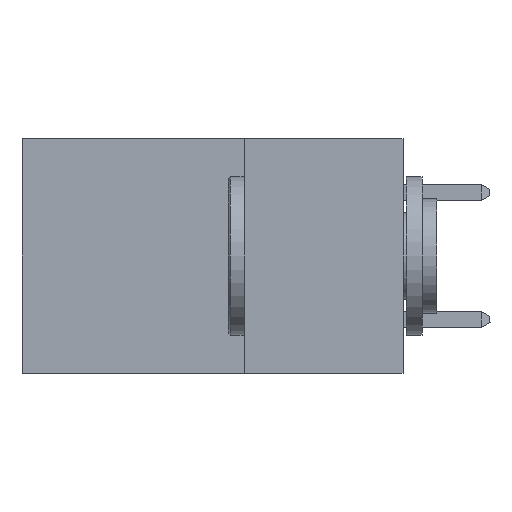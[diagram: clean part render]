
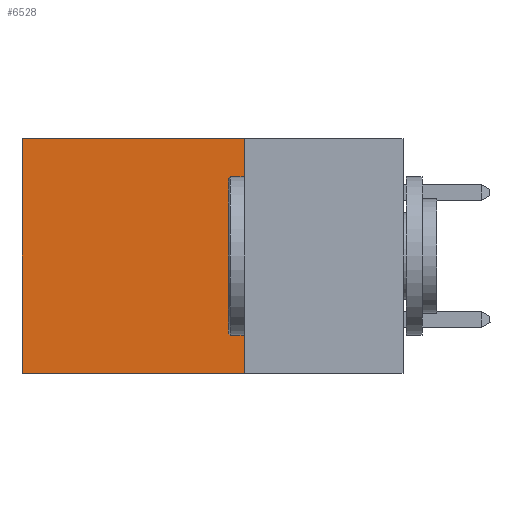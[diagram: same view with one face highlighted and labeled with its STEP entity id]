
A CAD part, left-side view. The second image highlights one B-rep face of the part: STEP entity #6528.
In plain terms, the highlighted planar face has unit normal (-1, 0, 0).
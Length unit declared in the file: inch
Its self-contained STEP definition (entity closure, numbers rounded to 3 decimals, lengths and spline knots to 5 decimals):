
#82 = FACE_OUTER_BOUND ( 'NONE', #4745, .T. ) ;
#235 = EDGE_CURVE ( 'NONE', #3854, #10123, #16813, .T. ) ;
#1263 = CARTESIAN_POINT ( 'NONE',  ( 0.2875, 0.25, 0. ) ) ;
#1335 = CARTESIAN_POINT ( 'NONE',  ( 0.2875, 0.25, 0. ) ) ;
#2133 = VERTEX_POINT ( 'NONE', #13537 ) ;
#3616 = EDGE_CURVE ( 'NONE', #3854, #2133, #17326, .T. ) ;
#3746 = CARTESIAN_POINT ( 'NONE',  ( 0.2875, 0.25, 0. ) ) ;
#3851 = DIRECTION ( 'NONE',  ( 0., 0., -1. ) ) ;
#3854 = VERTEX_POINT ( 'NONE', #3746 ) ;
#4299 = EDGE_CURVE ( 'NONE', #2133, #10515, #11146, .T. ) ;
#4745 = EDGE_LOOP ( 'NONE', ( #16329, #11081, #9070, #13059 ) ) ;
#5751 = DIRECTION ( 'NONE',  ( 0., 1., 0. ) ) ;
#6263 = VECTOR ( 'NONE', #3851, 39.37008 ) ;
#6358 = CARTESIAN_POINT ( 'NONE',  ( 0.2875, 0.25, -0.37 ) ) ;
#6528 = ADVANCED_FACE ( 'NONE', ( #82 ), #13390, .F. ) ;
#6806 = DIRECTION ( 'NONE',  ( 0., 0., -1. ) ) ;
#6993 = CARTESIAN_POINT ( 'NONE',  ( 0.2875, 0.25, 0. ) ) ;
#7622 = VECTOR ( 'NONE', #8741, 39.37008 ) ;
#8685 = LINE ( 'NONE', #14033, #15696 ) ;
#8741 = DIRECTION ( 'NONE',  ( 0., 0., -1. ) ) ;
#9070 = ORIENTED_EDGE ( 'NONE', *, *, #235, .F. ) ;
#9808 = CARTESIAN_POINT ( 'NONE',  ( 0.2875, 0.6, -0.37 ) ) ;
#10123 = VERTEX_POINT ( 'NONE', #6358 ) ;
#10144 = DIRECTION ( 'NONE',  ( 0., 1., 0. ) ) ;
#10317 = VECTOR ( 'NONE', #5751, 39.37008 ) ;
#10515 = VERTEX_POINT ( 'NONE', #9808 ) ;
#11081 = ORIENTED_EDGE ( 'NONE', *, *, #13144, .F. ) ;
#11146 = LINE ( 'NONE', #16637, #7622 ) ;
#12437 = AXIS2_PLACEMENT_3D ( 'NONE', #1335, #14710, #6806 ) ;
#13059 = ORIENTED_EDGE ( 'NONE', *, *, #3616, .T. ) ;
#13144 = EDGE_CURVE ( 'NONE', #10123, #10515, #8685, .T. ) ;
#13390 = PLANE ( 'NONE',  #12437 ) ;
#13537 = CARTESIAN_POINT ( 'NONE',  ( 0.2875, 0.6, 0. ) ) ;
#14033 = CARTESIAN_POINT ( 'NONE',  ( 0.2875, 0.25, -0.37 ) ) ;
#14710 = DIRECTION ( 'NONE',  ( 1., 0., 0. ) ) ;
#15696 = VECTOR ( 'NONE', #10144, 39.37008 ) ;
#16329 = ORIENTED_EDGE ( 'NONE', *, *, #4299, .T. ) ;
#16637 = CARTESIAN_POINT ( 'NONE',  ( 0.2875, 0.6, 0. ) ) ;
#16813 = LINE ( 'NONE', #1263, #6263 ) ;
#17326 = LINE ( 'NONE', #6993, #10317 ) ;
